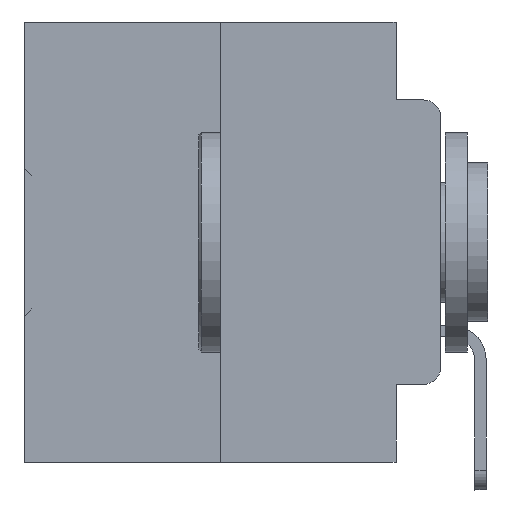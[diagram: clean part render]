
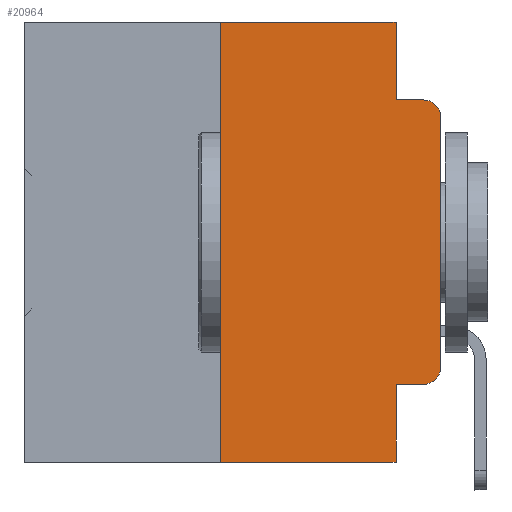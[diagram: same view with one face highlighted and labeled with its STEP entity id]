
A CAD part, left-side view. The second image highlights one B-rep face of the part: STEP entity #20964.
In plain terms, the highlighted planar face has unit normal (-1, 0, 0).
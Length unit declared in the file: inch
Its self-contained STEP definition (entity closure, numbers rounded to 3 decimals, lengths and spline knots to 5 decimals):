
#176 = ORIENTED_EDGE ( 'NONE', *, *, #5846, .F. ) ;
#1202 = EDGE_CURVE ( 'NONE', #36548, #36554, #22641, .T. ) ;
#1440 = AXIS2_PLACEMENT_3D ( 'NONE', #33667, #7846, #19363 ) ;
#2223 = LINE ( 'NONE', #21809, #21432 ) ;
#2709 = ORIENTED_EDGE ( 'NONE', *, *, #18735, .T. ) ;
#2974 = VECTOR ( 'NONE', #26203, 39.37008 ) ;
#2978 = VERTEX_POINT ( 'NONE', #19248 ) ;
#3343 = LINE ( 'NONE', #27091, #21110 ) ;
#3363 = CARTESIAN_POINT ( 'NONE',  ( 0., 0.25, -0.5 ) ) ;
#3659 = CARTESIAN_POINT ( 'NONE',  ( 0., 0.051, -0.0885 ) ) ;
#3667 = ORIENTED_EDGE ( 'NONE', *, *, #31404, .F. ) ;
#4803 = CARTESIAN_POINT ( 'NONE',  ( 0., 0.051, 0. ) ) ;
#5844 = CARTESIAN_POINT ( 'NONE',  ( 0., 0.051, -0.0885 ) ) ;
#5846 = EDGE_CURVE ( 'NONE', #33250, #24409, #23776, .T. ) ;
#6985 = CARTESIAN_POINT ( 'NONE',  ( 0., 0.051, -0.4115 ) ) ;
#7313 = CARTESIAN_POINT ( 'NONE',  ( 0., 0.473, 0. ) ) ;
#7498 = DIRECTION ( 'NONE',  ( 1., 0., 0. ) ) ;
#7694 = FACE_OUTER_BOUND ( 'NONE', #24887, .T. ) ;
#7846 = DIRECTION ( 'NONE',  ( -1., 0., 0. ) ) ;
#7959 = DIRECTION ( 'NONE',  ( 0., -1., 0. ) ) ;
#8509 = VECTOR ( 'NONE', #7959, 39.37008 ) ;
#8673 = DIRECTION ( 'NONE',  ( 0., 0., -1. ) ) ;
#9821 = EDGE_CURVE ( 'NONE', #24409, #2978, #23631, .T. ) ;
#10630 = VECTOR ( 'NONE', #20638, 39.37008 ) ;
#11158 = CARTESIAN_POINT ( 'NONE',  ( 0., 0.051, -0.4115 ) ) ;
#11174 = CARTESIAN_POINT ( 'NONE',  ( 0., 0., -0.1085 ) ) ;
#11213 = EDGE_CURVE ( 'NONE', #2978, #30562, #32360, .T. ) ;
#11335 = ORIENTED_EDGE ( 'NONE', *, *, #25683, .T. ) ;
#11337 = LINE ( 'NONE', #11158, #8509 ) ;
#11995 = DIRECTION ( 'NONE',  ( 0., -1., 0. ) ) ;
#13213 = EDGE_CURVE ( 'NONE', #33250, #28942, #3343, .T. ) ;
#13540 = ORIENTED_EDGE ( 'NONE', *, *, #13213, .T. ) ;
#14335 = CARTESIAN_POINT ( 'NONE',  ( 0., 0.051, 0. ) ) ;
#14345 = ORIENTED_EDGE ( 'NONE', *, *, #11213, .F. ) ;
#14698 = LINE ( 'NONE', #5844, #2974 ) ;
#15797 = DIRECTION ( 'NONE',  ( 0., 0., -1. ) ) ;
#16091 = CARTESIAN_POINT ( 'NONE',  ( 0., 0.02, -0.3915 ) ) ;
#16788 = EDGE_CURVE ( 'NONE', #32910, #36548, #11337, .T. ) ;
#17242 = CARTESIAN_POINT ( 'NONE',  ( 0., 0.051, -0.5 ) ) ;
#17718 = LINE ( 'NONE', #14335, #21566 ) ;
#18735 = EDGE_CURVE ( 'NONE', #35366, #20397, #25494, .T. ) ;
#19214 = VECTOR ( 'NONE', #26805, 39.37008 ) ;
#19248 = CARTESIAN_POINT ( 'NONE',  ( 0., 0.051, 0. ) ) ;
#19363 = DIRECTION ( 'NONE',  ( 0., 0., -1. ) ) ;
#20397 = VERTEX_POINT ( 'NONE', #35280 ) ;
#20638 = DIRECTION ( 'NONE',  ( 0., -1., 0. ) ) ;
#20964 = ADVANCED_FACE ( 'NONE', ( #7694 ), #36319, .F. ) ;
#21110 = VECTOR ( 'NONE', #11995, 39.37008 ) ;
#21235 = AXIS2_PLACEMENT_3D ( 'NONE', #7313, #7498, #15797 ) ;
#21432 = VECTOR ( 'NONE', #22360, 39.37008 ) ;
#21566 = VECTOR ( 'NONE', #8673, 39.37008 ) ;
#21809 = CARTESIAN_POINT ( 'NONE',  ( 0., 0., 0. ) ) ;
#22360 = DIRECTION ( 'NONE',  ( 0., 0., 1. ) ) ;
#22641 = CIRCLE ( 'NONE', #34064, 0.02 ) ;
#23631 = LINE ( 'NONE', #26291, #10630 ) ;
#23776 = LINE ( 'NONE', #24149, #19214 ) ;
#24149 = CARTESIAN_POINT ( 'NONE',  ( 0., 0.25, 0. ) ) ;
#24409 = VERTEX_POINT ( 'NONE', #36943 ) ;
#24887 = EDGE_LOOP ( 'NONE', ( #11335, #2709, #26505, #14345, #29614, #176, #13540, #3667, #33550, #33468 ) ) ;
#25494 = CIRCLE ( 'NONE', #1440, 0.02 ) ;
#25683 = EDGE_CURVE ( 'NONE', #36554, #35366, #2223, .T. ) ;
#26203 = DIRECTION ( 'NONE',  ( 0., -1., 0. ) ) ;
#26291 = CARTESIAN_POINT ( 'NONE',  ( 0., 0.473, 0. ) ) ;
#26505 = ORIENTED_EDGE ( 'NONE', *, *, #35862, .F. ) ;
#26805 = DIRECTION ( 'NONE',  ( 0., 0., 1. ) ) ;
#27091 = CARTESIAN_POINT ( 'NONE',  ( 0., 0.473, -0.5 ) ) ;
#27946 = DIRECTION ( 'NONE',  ( 0., 0., -1. ) ) ;
#28306 = DIRECTION ( 'NONE',  ( -1., 0., 0. ) ) ;
#28942 = VERTEX_POINT ( 'NONE', #17242 ) ;
#29614 = ORIENTED_EDGE ( 'NONE', *, *, #9821, .F. ) ;
#30093 = CARTESIAN_POINT ( 'NONE',  ( 0., 0.02, -0.4115 ) ) ;
#30562 = VERTEX_POINT ( 'NONE', #3659 ) ;
#31404 = EDGE_CURVE ( 'NONE', #32910, #28942, #17718, .T. ) ;
#32360 = LINE ( 'NONE', #4803, #35760 ) ;
#32910 = VERTEX_POINT ( 'NONE', #6985 ) ;
#33243 = DIRECTION ( 'NONE',  ( 0., 0., -1. ) ) ;
#33250 = VERTEX_POINT ( 'NONE', #3363 ) ;
#33468 = ORIENTED_EDGE ( 'NONE', *, *, #1202, .T. ) ;
#33550 = ORIENTED_EDGE ( 'NONE', *, *, #16788, .T. ) ;
#33667 = CARTESIAN_POINT ( 'NONE',  ( 0., 0.02, -0.1085 ) ) ;
#34064 = AXIS2_PLACEMENT_3D ( 'NONE', #16091, #28306, #27946 ) ;
#35280 = CARTESIAN_POINT ( 'NONE',  ( 0., 0.02, -0.0885 ) ) ;
#35366 = VERTEX_POINT ( 'NONE', #11174 ) ;
#35721 = CARTESIAN_POINT ( 'NONE',  ( 0., 0., -0.3915 ) ) ;
#35760 = VECTOR ( 'NONE', #33243, 39.37008 ) ;
#35862 = EDGE_CURVE ( 'NONE', #30562, #20397, #14698, .T. ) ;
#36319 = PLANE ( 'NONE',  #21235 ) ;
#36548 = VERTEX_POINT ( 'NONE', #30093 ) ;
#36554 = VERTEX_POINT ( 'NONE', #35721 ) ;
#36943 = CARTESIAN_POINT ( 'NONE',  ( 0., 0.25, 0. ) ) ;
